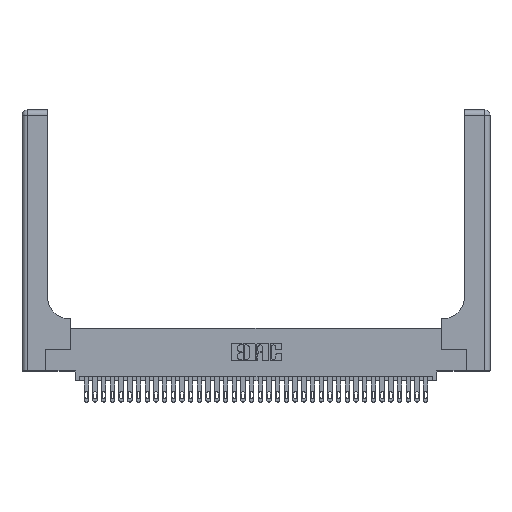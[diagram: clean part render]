
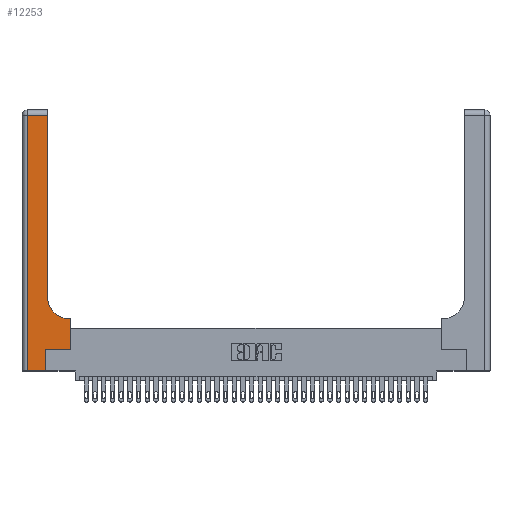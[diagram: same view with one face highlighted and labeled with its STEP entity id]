
A CAD part, top view. The second image highlights one B-rep face of the part: STEP entity #12253.
In plain terms, the highlighted planar face has unit normal (0, 0, 1).
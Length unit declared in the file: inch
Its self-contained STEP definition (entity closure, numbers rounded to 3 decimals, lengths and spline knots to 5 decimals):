
#43 = VECTOR ( 'NONE', #6667, 39.37008 ) ;
#1052 = DIRECTION ( 'NONE',  ( 0., 0., -1. ) ) ;
#1518 = EDGE_LOOP ( 'NONE', ( #34110, #6982, #15253, #10834, #34615, #21346, #6492, #31639, #11149 ) ) ;
#1538 = DIRECTION ( 'NONE',  ( 0., 1., 0. ) ) ;
#2478 = DIRECTION ( 'NONE',  ( -1., 0., 0. ) ) ;
#3030 = CARTESIAN_POINT ( 'NONE',  ( 0.5585, 0.6, 0.37 ) ) ;
#3162 = VECTOR ( 'NONE', #23621, 39.37008 ) ;
#3548 = EDGE_CURVE ( 'NONE', #20124, #36497, #26759, .T. ) ;
#3711 = EDGE_CURVE ( 'NONE', #26284, #24202, #4959, .T. ) ;
#4912 = CARTESIAN_POINT ( 'NONE',  ( 0.269, 0.25, 0.37 ) ) ;
#4959 = LINE ( 'NONE', #32944, #26307 ) ;
#5296 = CARTESIAN_POINT ( 'NONE',  ( 0.2915, 2.94, 0.37 ) ) ;
#5399 = LINE ( 'NONE', #29286, #34740 ) ;
#6070 = VECTOR ( 'NONE', #15959, 39.37008 ) ;
#6492 = ORIENTED_EDGE ( 'NONE', *, *, #25979, .T. ) ;
#6667 = DIRECTION ( 'NONE',  ( -1., 0., 0. ) ) ;
#6913 = PLANE ( 'NONE',  #22106 ) ;
#6982 = ORIENTED_EDGE ( 'NONE', *, *, #36752, .T. ) ;
#7580 = LINE ( 'NONE', #22943, #43 ) ;
#8486 = CARTESIAN_POINT ( 'NONE',  ( 0.269, 0., 0.37 ) ) ;
#9088 = LINE ( 'NONE', #22682, #24294 ) ;
#9544 = FACE_OUTER_BOUND ( 'NONE', #1518, .T. ) ;
#10084 = CARTESIAN_POINT ( 'NONE',  ( 0.5585, 0.25, 0.37 ) ) ;
#10273 = CARTESIAN_POINT ( 'NONE',  ( 0.06, 0., 0.37 ) ) ;
#10834 = ORIENTED_EDGE ( 'NONE', *, *, #30328, .T. ) ;
#11149 = ORIENTED_EDGE ( 'NONE', *, *, #36759, .T. ) ;
#11373 = VERTEX_POINT ( 'NONE', #35811 ) ;
#11833 = VERTEX_POINT ( 'NONE', #18899 ) ;
#12253 = ADVANCED_FACE ( 'NONE', ( #9544 ), #6913, .F. ) ;
#13816 = DIRECTION ( 'NONE',  ( 0., 0., -1. ) ) ;
#14298 = DIRECTION ( 'NONE',  ( 0., -1., 0. ) ) ;
#14313 = LINE ( 'NONE', #20370, #3162 ) ;
#14571 = EDGE_CURVE ( 'NONE', #33598, #23259, #14313, .T. ) ;
#15133 = DIRECTION ( 'NONE',  ( 1., 0., 0. ) ) ;
#15253 = ORIENTED_EDGE ( 'NONE', *, *, #20202, .T. ) ;
#15959 = DIRECTION ( 'NONE',  ( 0., 1., 0. ) ) ;
#16256 = VECTOR ( 'NONE', #18392, 39.37008 ) ;
#17775 = DIRECTION ( 'NONE',  ( 1., 0., 0. ) ) ;
#18392 = DIRECTION ( 'NONE',  ( 1., 0., 0. ) ) ;
#18899 = CARTESIAN_POINT ( 'NONE',  ( 0.5585, 0.25, 0.37 ) ) ;
#20124 = VERTEX_POINT ( 'NONE', #27232 ) ;
#20129 = VERTEX_POINT ( 'NONE', #10273 ) ;
#20202 = EDGE_CURVE ( 'NONE', #11373, #20129, #9088, .T. ) ;
#20370 = CARTESIAN_POINT ( 'NONE',  ( 0.2915, 0.6, 0.37 ) ) ;
#21346 = ORIENTED_EDGE ( 'NONE', *, *, #33779, .T. ) ;
#21851 = CIRCLE ( 'NONE', #34307, 0.25 ) ;
#22106 = AXIS2_PLACEMENT_3D ( 'NONE', #27896, #13816, #2478 ) ;
#22597 = LINE ( 'NONE', #10084, #6070 ) ;
#22682 = CARTESIAN_POINT ( 'NONE',  ( 0.06, 3., 0.37 ) ) ;
#22943 = CARTESIAN_POINT ( 'NONE',  ( 0., 2.94, 0.37 ) ) ;
#23259 = VERTEX_POINT ( 'NONE', #33305 ) ;
#23621 = DIRECTION ( 'NONE',  ( -1., 0., 0. ) ) ;
#24202 = VERTEX_POINT ( 'NONE', #4912 ) ;
#24294 = VECTOR ( 'NONE', #14298, 39.37008 ) ;
#25061 = VECTOR ( 'NONE', #1538, 39.37008 ) ;
#25979 = EDGE_CURVE ( 'NONE', #11833, #33598, #22597, .T. ) ;
#26284 = VERTEX_POINT ( 'NONE', #8486 ) ;
#26307 = VECTOR ( 'NONE', #30218, 39.37008 ) ;
#26759 = LINE ( 'NONE', #33076, #25061 ) ;
#27232 = CARTESIAN_POINT ( 'NONE',  ( 0.2915, 0.85, 0.37 ) ) ;
#27896 = CARTESIAN_POINT ( 'NONE',  ( 0., 3., 0.37 ) ) ;
#29286 = CARTESIAN_POINT ( 'NONE',  ( 0., 0., 0.37 ) ) ;
#30102 = LINE ( 'NONE', #31894, #16256 ) ;
#30218 = DIRECTION ( 'NONE',  ( 0., 1., 0. ) ) ;
#30328 = EDGE_CURVE ( 'NONE', #20129, #26284, #5399, .T. ) ;
#31639 = ORIENTED_EDGE ( 'NONE', *, *, #14571, .T. ) ;
#31894 = CARTESIAN_POINT ( 'NONE',  ( 0.269, 0.25, 0.37 ) ) ;
#32003 = CARTESIAN_POINT ( 'NONE',  ( 0.5415, 0.85, 0.37 ) ) ;
#32944 = CARTESIAN_POINT ( 'NONE',  ( 0.269, 0., 0.37 ) ) ;
#33076 = CARTESIAN_POINT ( 'NONE',  ( 0.2915, 3., 0.37 ) ) ;
#33305 = CARTESIAN_POINT ( 'NONE',  ( 0.5415, 0.6, 0.37 ) ) ;
#33598 = VERTEX_POINT ( 'NONE', #3030 ) ;
#33779 = EDGE_CURVE ( 'NONE', #24202, #11833, #30102, .T. ) ;
#34110 = ORIENTED_EDGE ( 'NONE', *, *, #3548, .T. ) ;
#34307 = AXIS2_PLACEMENT_3D ( 'NONE', #32003, #1052, #15133 ) ;
#34615 = ORIENTED_EDGE ( 'NONE', *, *, #3711, .T. ) ;
#34740 = VECTOR ( 'NONE', #17775, 39.37008 ) ;
#35811 = CARTESIAN_POINT ( 'NONE',  ( 0.06, 2.94, 0.37 ) ) ;
#36497 = VERTEX_POINT ( 'NONE', #5296 ) ;
#36752 = EDGE_CURVE ( 'NONE', #36497, #11373, #7580, .T. ) ;
#36759 = EDGE_CURVE ( 'NONE', #23259, #20124, #21851, .T. ) ;
